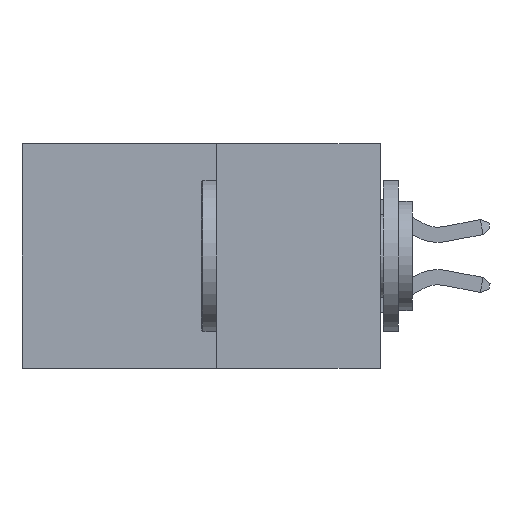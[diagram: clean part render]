
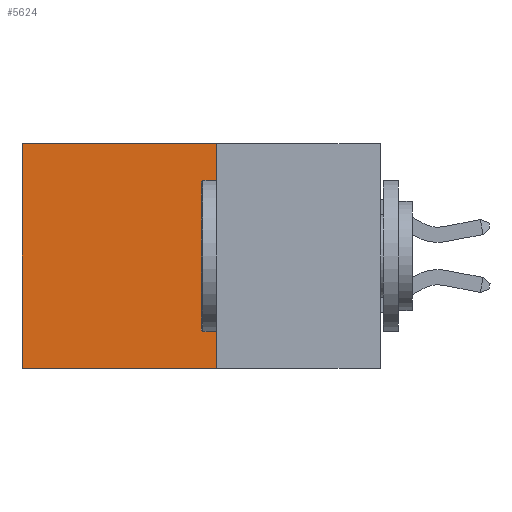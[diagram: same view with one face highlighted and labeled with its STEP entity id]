
A CAD part, left-side view. The second image highlights one B-rep face of the part: STEP entity #5624.
In plain terms, the highlighted planar face has unit normal (-1, 0, 0).
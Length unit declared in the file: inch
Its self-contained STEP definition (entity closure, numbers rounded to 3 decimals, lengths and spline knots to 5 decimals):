
#41 = EDGE_CURVE ( 'NONE', #12501, #11291, #12799, .T. ) ;
#781 = EDGE_CURVE ( 'NONE', #12501, #6015, #13092, .T. ) ;
#868 = LINE ( 'NONE', #4877, #10245 ) ;
#1364 = AXIS2_PLACEMENT_3D ( 'NONE', #6223, #1418, #9619 ) ;
#1418 = DIRECTION ( 'NONE',  ( 1., 0., 0. ) ) ;
#2037 = CARTESIAN_POINT ( 'NONE',  ( 0.277, 0.27, -0.37 ) ) ;
#3325 = CARTESIAN_POINT ( 'NONE',  ( 0.277, 0.27, -0.37 ) ) ;
#3370 = DIRECTION ( 'NONE',  ( 0., 1., 0. ) ) ;
#4030 = CARTESIAN_POINT ( 'NONE',  ( 0.277, 0.27, 0. ) ) ;
#4184 = CARTESIAN_POINT ( 'NONE',  ( 0.277, 0.27, 0. ) ) ;
#4425 = ORIENTED_EDGE ( 'NONE', *, *, #781, .F. ) ;
#4698 = EDGE_CURVE ( 'NONE', #11291, #8696, #868, .T. ) ;
#4877 = CARTESIAN_POINT ( 'NONE',  ( 0.277, 0.59, -0.37 ) ) ;
#5624 = ADVANCED_FACE ( 'NONE', ( #12653 ), #8487, .F. ) ;
#5754 = CARTESIAN_POINT ( 'NONE',  ( 0.277, 0.27, -0.37 ) ) ;
#6015 = VERTEX_POINT ( 'NONE', #3325 ) ;
#6223 = CARTESIAN_POINT ( 'NONE',  ( 0.277, 0.27, -0.37 ) ) ;
#6824 = VECTOR ( 'NONE', #9578, 39.37008 ) ;
#6979 = ORIENTED_EDGE ( 'NONE', *, *, #4698, .T. ) ;
#7560 = VECTOR ( 'NONE', #7884, 39.37008 ) ;
#7836 = ORIENTED_EDGE ( 'NONE', *, *, #41, .T. ) ;
#7884 = DIRECTION ( 'NONE',  ( 0., 1., 0. ) ) ;
#8255 = DIRECTION ( 'NONE',  ( 0., 0., -1. ) ) ;
#8487 = PLANE ( 'NONE',  #1364 ) ;
#8696 = VERTEX_POINT ( 'NONE', #14066 ) ;
#9578 = DIRECTION ( 'NONE',  ( 0., 0., -1. ) ) ;
#9619 = DIRECTION ( 'NONE',  ( 0., 0., -1. ) ) ;
#9860 = VECTOR ( 'NONE', #3370, 39.37008 ) ;
#10245 = VECTOR ( 'NONE', #8255, 39.37008 ) ;
#10749 = ORIENTED_EDGE ( 'NONE', *, *, #12717, .F. ) ;
#10929 = LINE ( 'NONE', #2037, #7560 ) ;
#11291 = VERTEX_POINT ( 'NONE', #13227 ) ;
#12501 = VERTEX_POINT ( 'NONE', #4184 ) ;
#12653 = FACE_OUTER_BOUND ( 'NONE', #14242, .T. ) ;
#12717 = EDGE_CURVE ( 'NONE', #6015, #8696, #10929, .T. ) ;
#12799 = LINE ( 'NONE', #4030, #9860 ) ;
#13092 = LINE ( 'NONE', #5754, #6824 ) ;
#13227 = CARTESIAN_POINT ( 'NONE',  ( 0.277, 0.59, 0. ) ) ;
#14066 = CARTESIAN_POINT ( 'NONE',  ( 0.277, 0.59, -0.37 ) ) ;
#14242 = EDGE_LOOP ( 'NONE', ( #6979, #10749, #4425, #7836 ) ) ;
